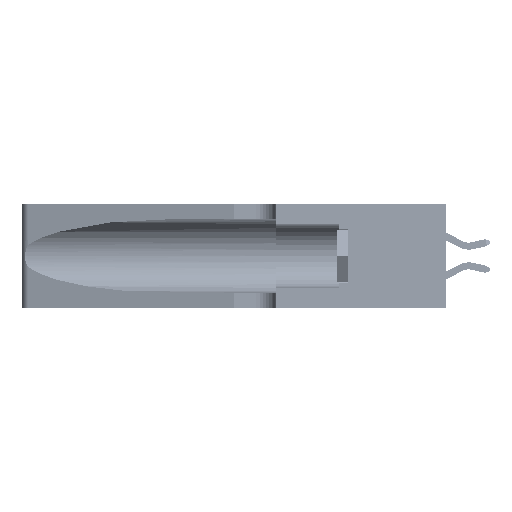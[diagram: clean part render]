
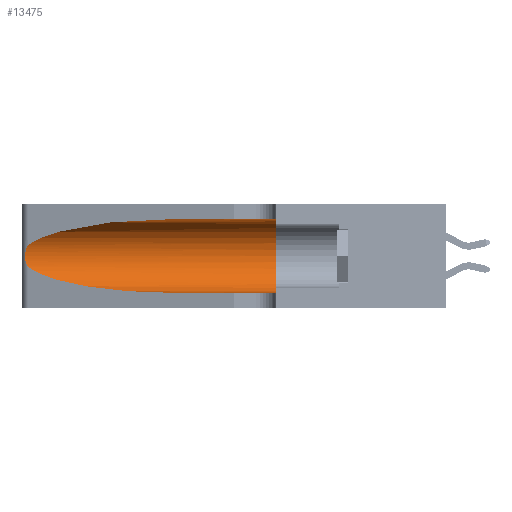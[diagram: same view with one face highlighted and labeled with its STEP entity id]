
A CAD part, left-side view. The second image highlights one B-rep face of the part: STEP entity #13475.
In plain terms, the highlighted cylindrical face has radius 3.308 mm (diameter 6.617 mm), a partial arc.
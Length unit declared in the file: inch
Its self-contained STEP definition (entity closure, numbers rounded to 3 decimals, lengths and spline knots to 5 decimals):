
#1121 = ORIENTED_EDGE ( 'NONE', *, *, #41965, .T. ) ;
#1158 = CARTESIAN_POINT ( 'NONE',  ( 0.25555, 1.22993, 0.14849 ) ) ;
#2952 = CIRCLE ( 'NONE', #44063, 0.13025 ) ;
#3499 = CARTESIAN_POINT ( 'NONE',  ( 0.25487, 1.22718, 0.14631 ) ) ;
#3854 = LINE ( 'NONE', #43484, #26887 ) ;
#3944 = CARTESIAN_POINT ( 'NONE',  ( 0.2373, 1.15595, 0.28018 ) ) ;
#4055 = VERTEX_POINT ( 'NONE', #32268 ) ;
#4562 = CARTESIAN_POINT ( 'NONE',  ( 0.25639, 1.23186, 0.15144 ) ) ;
#6060 = B_SPLINE_CURVE_WITH_KNOTS ( 'NONE', 3,
 ( #43627, #25741, #18631, #32952, #15044, #44083, #36714, #18317, #11463, #11299, #36567, #4562, #1158, #29213 ),
 .UNSPECIFIED., .F., .F.,
 ( 4, 2, 2, 2, 2, 2, 4 ),
 ( 0., 0.00027, 0.00053, 0.00107, 0.0016, 0.00187, 0.00214 ),
 .UNSPECIFIED. ) ;
#6445 = CARTESIAN_POINT ( 'NONE',  ( 0.1305, 0.35, 0.31525 ) ) ;
#6961 = DIRECTION ( 'NONE',  ( 0., 0., -1. ) ) ;
#8115 = EDGE_CURVE ( 'NONE', #37671, #44323, #6060, .T. ) ;
#8294 =( BOUNDED_CURVE ( )  B_SPLINE_CURVE ( 3, ( #3499, #13674, #42555, #13820 ),
 .UNSPECIFIED., .F., .T. ) 
 B_SPLINE_CURVE_WITH_KNOTS ( ( 4, 4 ),
 ( 3.44316, 4.71239 ),
 .UNSPECIFIED. ) 
 CURVE ( )  GEOMETRIC_REPRESENTATION_ITEM ( )  RATIONAL_B_SPLINE_CURVE ( ( 1., 0.87, 0.87, 1. ) ) 
 REPRESENTATION_ITEM ( '' )  );
#8887 =( BOUNDED_CURVE ( )  B_SPLINE_CURVE ( 3, ( #43011, #21765, #3944, #32361 ),
 .UNSPECIFIED., .F., .F. ) 
 B_SPLINE_CURVE_WITH_KNOTS ( ( 4, 4 ),
 ( 1.5708, 2.84003 ),
 .UNSPECIFIED. ) 
 CURVE ( )  GEOMETRIC_REPRESENTATION_ITEM ( )  RATIONAL_B_SPLINE_CURVE ( ( 1., 0.87, 0.87, 1. ) ) 
 REPRESENTATION_ITEM ( '' )  );
#9224 = LINE ( 'NONE', #12377, #17604 ) ;
#10141 = AXIS2_PLACEMENT_3D ( 'NONE', #24951, #28582, #6961 ) ;
#10834 = EDGE_CURVE ( 'NONE', #4055, #23171, #3854, .T. ) ;
#11299 = CARTESIAN_POINT ( 'NONE',  ( 0.25856, 1.23593, 0.16098 ) ) ;
#11463 = CARTESIAN_POINT ( 'NONE',  ( 0.26017, 1.23833, 0.17102 ) ) ;
#11515 = ORIENTED_EDGE ( 'NONE', *, *, #14327, .F. ) ;
#12377 = CARTESIAN_POINT ( 'NONE',  ( 0.1305, 1.61858, 0.05475 ) ) ;
#13475 = ADVANCED_FACE ( 'NONE', ( #32671 ), #23068, .F. ) ;
#13487 = EDGE_CURVE ( 'NONE', #44323, #34710, #8294, .T. ) ;
#13674 = CARTESIAN_POINT ( 'NONE',  ( 0.2373, 1.15595, 0.08982 ) ) ;
#13820 = CARTESIAN_POINT ( 'NONE',  ( 0.1305, 0.72297, 0.05475 ) ) ;
#14327 = EDGE_CURVE ( 'NONE', #23171, #42445, #2952, .T. ) ;
#14775 = CARTESIAN_POINT ( 'NONE',  ( 0.25487, 1.22718, 0.14631 ) ) ;
#15044 = CARTESIAN_POINT ( 'NONE',  ( 0.25854, 1.2359, 0.20912 ) ) ;
#17604 = VECTOR ( 'NONE', #30621, 39.37008 ) ;
#17762 = ORIENTED_EDGE ( 'NONE', *, *, #13487, .T. ) ;
#18317 = CARTESIAN_POINT ( 'NONE',  ( 0.26075, 1.23896, 0.178 ) ) ;
#18631 = CARTESIAN_POINT ( 'NONE',  ( 0.25639, 1.23184, 0.21858 ) ) ;
#21148 = ORIENTED_EDGE ( 'NONE', *, *, #34061, .T. ) ;
#21310 = CARTESIAN_POINT ( 'NONE',  ( 0.1305, 0.72297, 0.05475 ) ) ;
#21765 = CARTESIAN_POINT ( 'NONE',  ( 0.18966, 0.96281, 0.31525 ) ) ;
#22168 = CARTESIAN_POINT ( 'NONE',  ( 0.1305, 0.35, 0.185 ) ) ;
#23068 = CYLINDRICAL_SURFACE ( 'NONE', #10141, 0.13025 ) ;
#23171 = VERTEX_POINT ( 'NONE', #6445 ) ;
#24517 = ORIENTED_EDGE ( 'NONE', *, *, #8115, .T. ) ;
#24546 = EDGE_LOOP ( 'NONE', ( #1121, #24517, #17762, #21148, #11515, #33540 ) ) ;
#24951 = CARTESIAN_POINT ( 'NONE',  ( 0.1305, 1.61858, 0.185 ) ) ;
#25741 = CARTESIAN_POINT ( 'NONE',  ( 0.25555, 1.22994, 0.2215 ) ) ;
#26887 = VECTOR ( 'NONE', #32951, 39.37008 ) ;
#28582 = DIRECTION ( 'NONE',  ( 0., -1., 0. ) ) ;
#29213 = CARTESIAN_POINT ( 'NONE',  ( 0.25487, 1.22718, 0.14631 ) ) ;
#30621 = DIRECTION ( 'NONE',  ( 0., -1., 0. ) ) ;
#32268 = CARTESIAN_POINT ( 'NONE',  ( 0.1305, 0.72297, 0.31525 ) ) ;
#32361 = CARTESIAN_POINT ( 'NONE',  ( 0.25487, 1.22718, 0.22369 ) ) ;
#32610 = DIRECTION ( 'NONE',  ( 0., 1., 0. ) ) ;
#32671 = FACE_OUTER_BOUND ( 'NONE', #24546, .T. ) ;
#32951 = DIRECTION ( 'NONE',  ( 0., -1., 0. ) ) ;
#32952 = CARTESIAN_POINT ( 'NONE',  ( 0.25787, 1.23484, 0.2124 ) ) ;
#33540 = ORIENTED_EDGE ( 'NONE', *, *, #10834, .F. ) ;
#34061 = EDGE_CURVE ( 'NONE', #34710, #42445, #9224, .T. ) ;
#34710 = VERTEX_POINT ( 'NONE', #21310 ) ;
#34881 = CARTESIAN_POINT ( 'NONE',  ( 0.25487, 1.22718, 0.22369 ) ) ;
#36567 = CARTESIAN_POINT ( 'NONE',  ( 0.25789, 1.23486, 0.15765 ) ) ;
#36714 = CARTESIAN_POINT ( 'NONE',  ( 0.26075, 1.23896, 0.19203 ) ) ;
#37671 = VERTEX_POINT ( 'NONE', #34881 ) ;
#38242 = CARTESIAN_POINT ( 'NONE',  ( 0.1305, 0.35, 0.05475 ) ) ;
#40113 = DIRECTION ( 'NONE',  ( 0., 0., 1. ) ) ;
#41965 = EDGE_CURVE ( 'NONE', #4055, #37671, #8887, .T. ) ;
#42445 = VERTEX_POINT ( 'NONE', #38242 ) ;
#42555 = CARTESIAN_POINT ( 'NONE',  ( 0.18966, 0.96281, 0.05475 ) ) ;
#43011 = CARTESIAN_POINT ( 'NONE',  ( 0.1305, 0.72297, 0.31525 ) ) ;
#43484 = CARTESIAN_POINT ( 'NONE',  ( 0.1305, 1.61858, 0.31525 ) ) ;
#43627 = CARTESIAN_POINT ( 'NONE',  ( 0.25487, 1.22718, 0.22369 ) ) ;
#44063 = AXIS2_PLACEMENT_3D ( 'NONE', #22168, #32610, #40113 ) ;
#44083 = CARTESIAN_POINT ( 'NONE',  ( 0.26018, 1.23835, 0.19895 ) ) ;
#44323 = VERTEX_POINT ( 'NONE', #14775 ) ;
